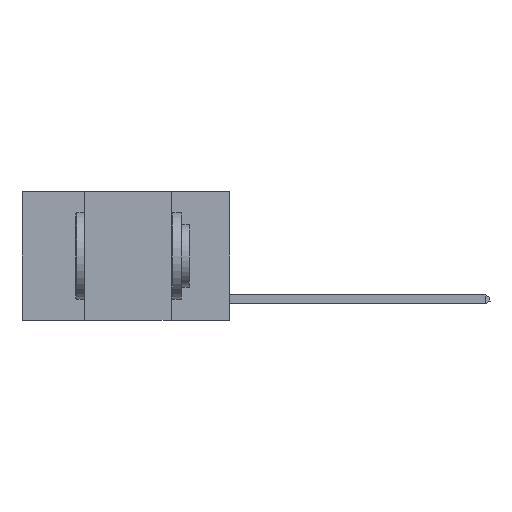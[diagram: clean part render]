
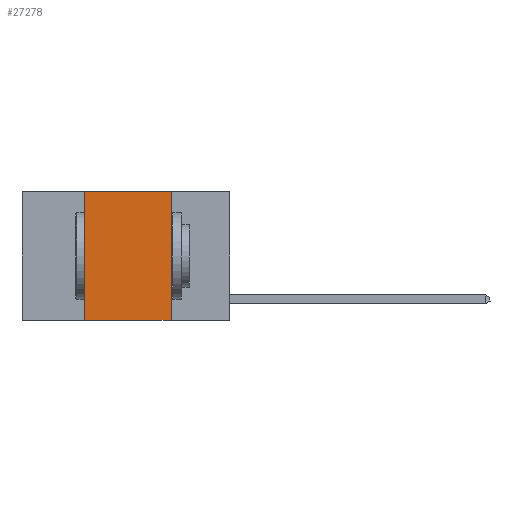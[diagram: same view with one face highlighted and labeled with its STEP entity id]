
A CAD part, left-side view. The second image highlights one B-rep face of the part: STEP entity #27278.
In plain terms, the highlighted planar face has unit normal (-1, 0, 0).
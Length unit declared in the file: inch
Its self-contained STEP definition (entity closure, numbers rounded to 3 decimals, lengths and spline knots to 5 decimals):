
#257 = ORIENTED_EDGE ( 'NONE', *, *, #18288, .F. ) ;
#864 = ORIENTED_EDGE ( 'NONE', *, *, #9673, .T. ) ;
#1606 = ORIENTED_EDGE ( 'NONE', *, *, #15432, .F. ) ;
#2701 = DIRECTION ( 'NONE',  ( 1., 0., 0. ) ) ;
#3258 = VERTEX_POINT ( 'NONE', #27323 ) ;
#3799 = CARTESIAN_POINT ( 'NONE',  ( 0., 0.17, 0. ) ) ;
#4422 = CARTESIAN_POINT ( 'NONE',  ( 0., 0.17, 0. ) ) ;
#5243 = ORIENTED_EDGE ( 'NONE', *, *, #20518, .F. ) ;
#7604 = VERTEX_POINT ( 'NONE', #21292 ) ;
#7694 = CARTESIAN_POINT ( 'NONE',  ( 0., 0.6, 0. ) ) ;
#9151 = VERTEX_POINT ( 'NONE', #3799 ) ;
#9528 = VECTOR ( 'NONE', #20637, 39.37008 ) ;
#9673 = EDGE_CURVE ( 'NONE', #24305, #7604, #26619, .T. ) ;
#12545 = LINE ( 'NONE', #16036, #23251 ) ;
#13282 = FACE_OUTER_BOUND ( 'NONE', #20035, .T. ) ;
#15432 = EDGE_CURVE ( 'NONE', #24305, #3258, #12545, .T. ) ;
#15585 = PLANE ( 'NONE',  #17784 ) ;
#16016 = VECTOR ( 'NONE', #18371, 39.37008 ) ;
#16036 = CARTESIAN_POINT ( 'NONE',  ( 0., 0.42, 0. ) ) ;
#17731 = DIRECTION ( 'NONE',  ( 0., 0., -1. ) ) ;
#17784 = AXIS2_PLACEMENT_3D ( 'NONE', #21910, #2701, #17731 ) ;
#18288 = EDGE_CURVE ( 'NONE', #9151, #7604, #23117, .T. ) ;
#18371 = DIRECTION ( 'NONE',  ( 0., -1., 0. ) ) ;
#18500 = CARTESIAN_POINT ( 'NONE',  ( 0., 0.6, -0.37 ) ) ;
#20035 = EDGE_LOOP ( 'NONE', ( #257, #5243, #1606, #864 ) ) ;
#20242 = DIRECTION ( 'NONE',  ( 0., 0., 1. ) ) ;
#20518 = EDGE_CURVE ( 'NONE', #3258, #9151, #27396, .T. ) ;
#20637 = DIRECTION ( 'NONE',  ( 0., -1., 0. ) ) ;
#21292 = CARTESIAN_POINT ( 'NONE',  ( 0., 0.17, -0.37 ) ) ;
#21910 = CARTESIAN_POINT ( 'NONE',  ( 0., 0.6, 0. ) ) ;
#22451 = VECTOR ( 'NONE', #25881, 39.37008 ) ;
#23117 = LINE ( 'NONE', #4422, #22451 ) ;
#23251 = VECTOR ( 'NONE', #20242, 39.37008 ) ;
#24305 = VERTEX_POINT ( 'NONE', #27529 ) ;
#25881 = DIRECTION ( 'NONE',  ( 0., 0., -1. ) ) ;
#26619 = LINE ( 'NONE', #18500, #9528 ) ;
#27278 = ADVANCED_FACE ( 'NONE', ( #13282 ), #15585, .F. ) ;
#27323 = CARTESIAN_POINT ( 'NONE',  ( 0., 0.42, 0. ) ) ;
#27396 = LINE ( 'NONE', #7694, #16016 ) ;
#27529 = CARTESIAN_POINT ( 'NONE',  ( 0., 0.42, -0.37 ) ) ;
